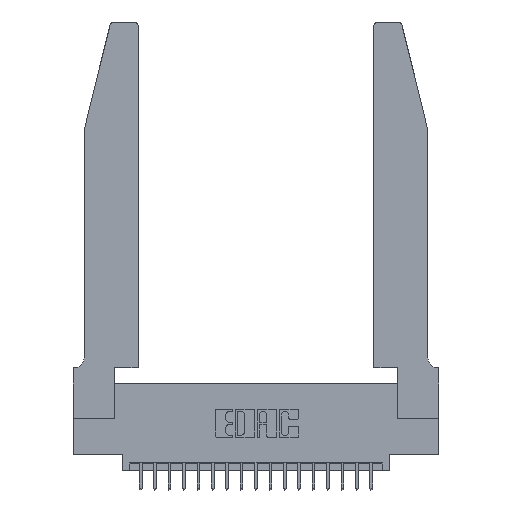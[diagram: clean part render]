
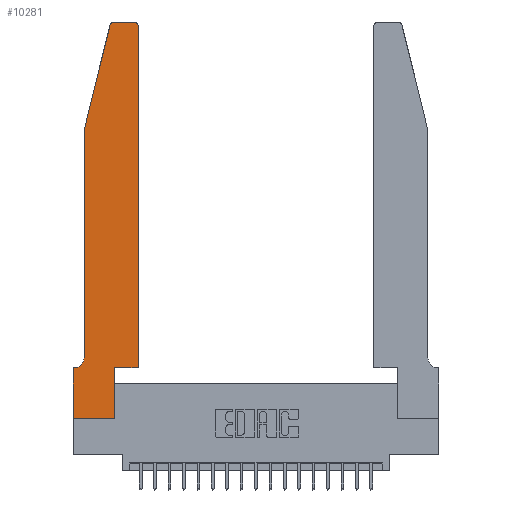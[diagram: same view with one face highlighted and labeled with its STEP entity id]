
A CAD part, top view. The second image highlights one B-rep face of the part: STEP entity #10281.
In plain terms, the highlighted planar face has unit normal (0, 0, 1).
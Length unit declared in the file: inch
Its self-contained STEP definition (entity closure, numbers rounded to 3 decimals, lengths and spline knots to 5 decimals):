
#76 = CARTESIAN_POINT ( 'NONE',  ( 0.4505, 2.72, 0.37 ) ) ;
#311 = CARTESIAN_POINT ( 'NONE',  ( 0.284, 2.72, 0.37 ) ) ;
#374 = DIRECTION ( 'NONE',  ( 1., 0., 0. ) ) ;
#505 = ORIENTED_EDGE ( 'NONE', *, *, #16784, .T. ) ;
#812 = VERTEX_POINT ( 'NONE', #15725 ) ;
#815 = VERTEX_POINT ( 'NONE', #5499 ) ;
#913 = VECTOR ( 'NONE', #21065, 39.37008 ) ;
#953 = CARTESIAN_POINT ( 'NONE',  ( 0.4205, 2.75, 0.37 ) ) ;
#1302 = CARTESIAN_POINT ( 'NONE',  ( 0.0055, 0.35, 0.37 ) ) ;
#1848 = CARTESIAN_POINT ( 'NONE',  ( 0.2865, 0.35, 0.37 ) ) ;
#1902 = VERTEX_POINT ( 'NONE', #14826 ) ;
#2235 = AXIS2_PLACEMENT_3D ( 'NONE', #19550, #16287, #6281 ) ;
#2392 = CARTESIAN_POINT ( 'NONE',  ( 0.0755, 2., 0.37 ) ) ;
#2550 = ORIENTED_EDGE ( 'NONE', *, *, #17753, .T. ) ;
#2598 = CARTESIAN_POINT ( 'NONE',  ( 0., 0., 0.37 ) ) ;
#3215 = LINE ( 'NONE', #14991, #10969 ) ;
#3378 = LINE ( 'NONE', #19740, #10145 ) ;
#3458 = AXIS2_PLACEMENT_3D ( 'NONE', #18914, #10810, #374 ) ;
#3611 = EDGE_CURVE ( 'NONE', #812, #12478, #18954, .T. ) ;
#3698 = AXIS2_PLACEMENT_3D ( 'NONE', #21502, #6589, #9667 ) ;
#3846 = EDGE_CURVE ( 'NONE', #12478, #18933, #19186, .T. ) ;
#3887 = VERTEX_POINT ( 'NONE', #11509 ) ;
#4406 = EDGE_CURVE ( 'NONE', #3887, #12752, #20893, .T. ) ;
#4615 = ORIENTED_EDGE ( 'NONE', *, *, #6966, .T. ) ;
#4820 = CARTESIAN_POINT ( 'NONE',  ( 0., 0.35, 0.37 ) ) ;
#4922 = DIRECTION ( 'NONE',  ( 0., -1., 0. ) ) ;
#4963 = EDGE_CURVE ( 'NONE', #12641, #812, #3215, .T. ) ;
#5499 = CARTESIAN_POINT ( 'NONE',  ( 0.0755, 0.42, 0.37 ) ) ;
#5548 = CARTESIAN_POINT ( 'NONE',  ( 0., 0., 0.37 ) ) ;
#5598 = ORIENTED_EDGE ( 'NONE', *, *, #8583, .T. ) ;
#5806 = CARTESIAN_POINT ( 'NONE',  ( 0., 0., 0.37 ) ) ;
#6256 = EDGE_LOOP ( 'NONE', ( #18987, #18191, #7440, #17015, #16045, #21359, #505, #4615, #2550, #5598, #20448, #21684 ) ) ;
#6281 = DIRECTION ( 'NONE',  ( 1., 0., 0. ) ) ;
#6414 = DIRECTION ( 'NONE',  ( -1., 0., 0. ) ) ;
#6589 = DIRECTION ( 'NONE',  ( 0., 0., -1. ) ) ;
#6966 = EDGE_CURVE ( 'NONE', #8500, #9644, #10055, .T. ) ;
#7021 = DIRECTION ( 'NONE',  ( 0., 0., 1. ) ) ;
#7440 = ORIENTED_EDGE ( 'NONE', *, *, #3846, .T. ) ;
#7447 = EDGE_CURVE ( 'NONE', #12752, #12641, #10670, .T. ) ;
#7811 = EDGE_CURVE ( 'NONE', #815, #12161, #12816, .T. ) ;
#7974 = VECTOR ( 'NONE', #18101, 39.37008 ) ;
#8120 = LINE ( 'NONE', #19951, #12866 ) ;
#8500 = VERTEX_POINT ( 'NONE', #5548 ) ;
#8583 = EDGE_CURVE ( 'NONE', #1902, #3887, #10526, .T. ) ;
#8795 = VECTOR ( 'NONE', #10845, 39.37008 ) ;
#8802 = AXIS2_PLACEMENT_3D ( 'NONE', #311, #7021, #10537 ) ;
#9054 = VERTEX_POINT ( 'NONE', #4820 ) ;
#9644 = VERTEX_POINT ( 'NONE', #19199 ) ;
#9667 = DIRECTION ( 'NONE',  ( -1., 0., 0. ) ) ;
#9730 = EDGE_CURVE ( 'NONE', #18933, #815, #3378, .T. ) ;
#9878 = VECTOR ( 'NONE', #10934, 39.37008 ) ;
#10055 = LINE ( 'NONE', #2598, #20799 ) ;
#10145 = VECTOR ( 'NONE', #4922, 39.37008 ) ;
#10281 = ADVANCED_FACE ( 'NONE', ( #20776 ), #15853, .T. ) ;
#10526 = LINE ( 'NONE', #14142, #8795 ) ;
#10537 = DIRECTION ( 'NONE',  ( 1., 0., 0. ) ) ;
#10670 = CIRCLE ( 'NONE', #2235, 0.03 ) ;
#10810 = DIRECTION ( 'NONE',  ( 0., 0., 1. ) ) ;
#10845 = DIRECTION ( 'NONE',  ( 1., 0., 0. ) ) ;
#10934 = DIRECTION ( 'NONE',  ( 0., 1., 0. ) ) ;
#10969 = VECTOR ( 'NONE', #6414, 39.37008 ) ;
#11509 = CARTESIAN_POINT ( 'NONE',  ( 0.4505, 0.35, 0.37 ) ) ;
#12161 = VERTEX_POINT ( 'NONE', #1302 ) ;
#12478 = VERTEX_POINT ( 'NONE', #15701 ) ;
#12641 = VERTEX_POINT ( 'NONE', #953 ) ;
#12752 = VERTEX_POINT ( 'NONE', #76 ) ;
#12816 = CIRCLE ( 'NONE', #3698, 0.07 ) ;
#12866 = VECTOR ( 'NONE', #18537, 39.37008 ) ;
#13237 = DIRECTION ( 'NONE',  ( 1., 0., 0. ) ) ;
#14142 = CARTESIAN_POINT ( 'NONE',  ( 0.4505, 0.35, 0.37 ) ) ;
#14826 = CARTESIAN_POINT ( 'NONE',  ( 0.2865, 0.35, 0.37 ) ) ;
#14991 = CARTESIAN_POINT ( 'NONE',  ( 0.2605, 2.75, 0.37 ) ) ;
#15701 = CARTESIAN_POINT ( 'NONE',  ( 0.25487, 2.72718, 0.37 ) ) ;
#15725 = CARTESIAN_POINT ( 'NONE',  ( 0.284, 2.75, 0.37 ) ) ;
#15737 = CARTESIAN_POINT ( 'NONE',  ( 0.0755, 2., 0.37 ) ) ;
#15811 = DIRECTION ( 'NONE',  ( -0.239, -0.971, 0. ) ) ;
#15853 = PLANE ( 'NONE',  #3458 ) ;
#16045 = ORIENTED_EDGE ( 'NONE', *, *, #7811, .T. ) ;
#16287 = DIRECTION ( 'NONE',  ( 0., 0., 1. ) ) ;
#16784 = EDGE_CURVE ( 'NONE', #9054, #8500, #17457, .T. ) ;
#16908 = LINE ( 'NONE', #1848, #7974 ) ;
#17015 = ORIENTED_EDGE ( 'NONE', *, *, #9730, .T. ) ;
#17457 = LINE ( 'NONE', #5806, #913 ) ;
#17588 = VECTOR ( 'NONE', #15811, 39.37008 ) ;
#17688 = EDGE_CURVE ( 'NONE', #12161, #9054, #8120, .T. ) ;
#17753 = EDGE_CURVE ( 'NONE', #9644, #1902, #16908, .T. ) ;
#18101 = DIRECTION ( 'NONE',  ( 0., 1., 0. ) ) ;
#18191 = ORIENTED_EDGE ( 'NONE', *, *, #3611, .T. ) ;
#18537 = DIRECTION ( 'NONE',  ( -1., 0., 0. ) ) ;
#18914 = CARTESIAN_POINT ( 'NONE',  ( 0., 0.35, 0.37 ) ) ;
#18933 = VERTEX_POINT ( 'NONE', #15737 ) ;
#18954 = CIRCLE ( 'NONE', #8802, 0.03 ) ;
#18987 = ORIENTED_EDGE ( 'NONE', *, *, #4963, .T. ) ;
#19186 = LINE ( 'NONE', #2392, #17588 ) ;
#19199 = CARTESIAN_POINT ( 'NONE',  ( 0.2865, 0., 0.37 ) ) ;
#19352 = CARTESIAN_POINT ( 'NONE',  ( 0.4505, 0.35, 0.37 ) ) ;
#19550 = CARTESIAN_POINT ( 'NONE',  ( 0.4205, 2.72, 0.37 ) ) ;
#19740 = CARTESIAN_POINT ( 'NONE',  ( 0.0755, 2., 0.37 ) ) ;
#19951 = CARTESIAN_POINT ( 'NONE',  ( 0.0755, 0.35, 0.37 ) ) ;
#20448 = ORIENTED_EDGE ( 'NONE', *, *, #4406, .T. ) ;
#20776 = FACE_OUTER_BOUND ( 'NONE', #6256, .T. ) ;
#20799 = VECTOR ( 'NONE', #13237, 39.37008 ) ;
#20893 = LINE ( 'NONE', #19352, #9878 ) ;
#21065 = DIRECTION ( 'NONE',  ( 0., -1., 0. ) ) ;
#21359 = ORIENTED_EDGE ( 'NONE', *, *, #17688, .T. ) ;
#21502 = CARTESIAN_POINT ( 'NONE',  ( 0.0055, 0.42, 0.37 ) ) ;
#21684 = ORIENTED_EDGE ( 'NONE', *, *, #7447, .T. ) ;
